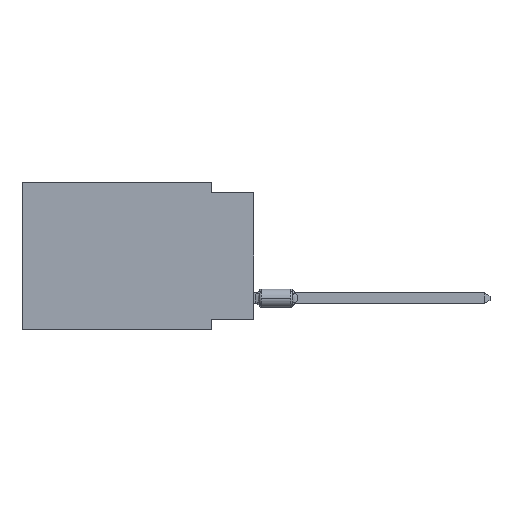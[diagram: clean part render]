
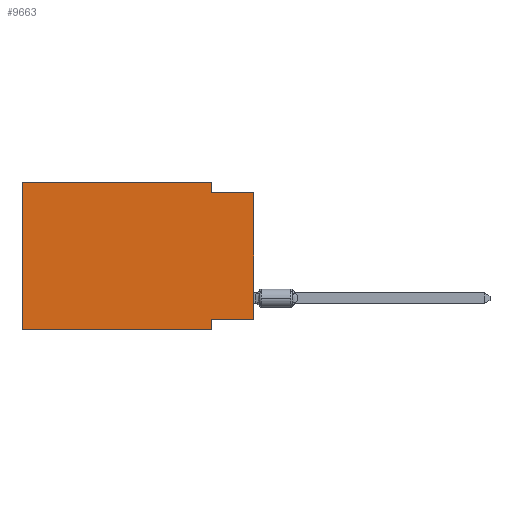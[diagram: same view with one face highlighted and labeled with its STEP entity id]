
A CAD part, left-side view. The second image highlights one B-rep face of the part: STEP entity #9663.
In plain terms, the highlighted planar face has unit normal (-1, 0, 0).
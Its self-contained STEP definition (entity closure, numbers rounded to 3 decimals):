
#119 = EDGE_CURVE ( 'NONE', #4076, #11084, #7150, .T. ) ;
#1149 = EDGE_CURVE ( 'NONE', #2157, #9634, #4121, .T. ) ;
#1265 = VECTOR ( 'NONE', #4323, 1000. ) ;
#1350 = DIRECTION ( 'NONE',  ( 0., 0., -1. ) ) ;
#1487 = LINE ( 'NONE', #12719, #3910 ) ;
#1554 = EDGE_CURVE ( 'NONE', #5131, #2082, #3403, .T. ) ;
#1648 = ORIENTED_EDGE ( 'NONE', *, *, #1554, .F. ) ;
#1771 = VECTOR ( 'NONE', #1350, 1000. ) ;
#2082 = VERTEX_POINT ( 'NONE', #5509 ) ;
#2157 = VERTEX_POINT ( 'NONE', #2670 ) ;
#2222 = ORIENTED_EDGE ( 'NONE', *, *, #9824, .T. ) ;
#2359 = ORIENTED_EDGE ( 'NONE', *, *, #119, .F. ) ;
#2578 = LINE ( 'NONE', #8451, #3247 ) ;
#2670 = CARTESIAN_POINT ( 'NONE',  ( 0., 13.97, -8.89 ) ) ;
#2773 = VECTOR ( 'NONE', #11607, 1000. ) ;
#3015 = ORIENTED_EDGE ( 'NONE', *, *, #6114, .F. ) ;
#3231 = LINE ( 'NONE', #10504, #1771 ) ;
#3247 = VECTOR ( 'NONE', #11606, 1000. ) ;
#3403 = LINE ( 'NONE', #7505, #2773 ) ;
#3701 = AXIS2_PLACEMENT_3D ( 'NONE', #9966, #6735, #7949 ) ;
#3910 = VECTOR ( 'NONE', #8354, 1000. ) ;
#4076 = VERTEX_POINT ( 'NONE', #4730 ) ;
#4086 = CARTESIAN_POINT ( 'NONE',  ( 0., 0., -8.255 ) ) ;
#4121 = LINE ( 'NONE', #11397, #1265 ) ;
#4323 = DIRECTION ( 'NONE',  ( 0., 0., 1. ) ) ;
#4683 = VECTOR ( 'NONE', #11817, 1000. ) ;
#4730 = CARTESIAN_POINT ( 'NONE',  ( 0., 2.54, -0.635 ) ) ;
#5131 = VERTEX_POINT ( 'NONE', #4086 ) ;
#5509 = CARTESIAN_POINT ( 'NONE',  ( 0., 2.54, -8.255 ) ) ;
#5958 = EDGE_CURVE ( 'NONE', #2157, #9488, #12956, .T. ) ;
#6114 = EDGE_CURVE ( 'NONE', #9634, #10293, #13154, .T. ) ;
#6343 = CARTESIAN_POINT ( 'NONE',  ( 0., 2.54, -8.89 ) ) ;
#6682 = ORIENTED_EDGE ( 'NONE', *, *, #1149, .F. ) ;
#6698 = ORIENTED_EDGE ( 'NONE', *, *, #9852, .F. ) ;
#6735 = DIRECTION ( 'NONE',  ( 1., 0., 0. ) ) ;
#7150 = LINE ( 'NONE', #8375, #8580 ) ;
#7209 = ORIENTED_EDGE ( 'NONE', *, *, #5958, .T. ) ;
#7229 = CARTESIAN_POINT ( 'NONE',  ( 0., 13.97, 0. ) ) ;
#7505 = CARTESIAN_POINT ( 'NONE',  ( 0., 0., -8.255 ) ) ;
#7733 = EDGE_LOOP ( 'NONE', ( #2222, #2359, #6698, #3015, #6682, #7209, #10249, #1648 ) ) ;
#7742 = FACE_OUTER_BOUND ( 'NONE', #7733, .T. ) ;
#7805 = CARTESIAN_POINT ( 'NONE',  ( 0., 13.97, 0. ) ) ;
#7949 = DIRECTION ( 'NONE',  ( 0., 0., -1. ) ) ;
#8354 = DIRECTION ( 'NONE',  ( 0., 0., 1. ) ) ;
#8375 = CARTESIAN_POINT ( 'NONE',  ( 0., 0., -0.635 ) ) ;
#8451 = CARTESIAN_POINT ( 'NONE',  ( 0., 2.54, -8.89 ) ) ;
#8580 = VECTOR ( 'NONE', #10448, 1000. ) ;
#8612 = EDGE_CURVE ( 'NONE', #2082, #9488, #2578, .T. ) ;
#8795 = CARTESIAN_POINT ( 'NONE',  ( 0., 2.54, 0. ) ) ;
#9488 = VERTEX_POINT ( 'NONE', #6343 ) ;
#9633 = VECTOR ( 'NONE', #10330, 1000. ) ;
#9634 = VERTEX_POINT ( 'NONE', #7805 ) ;
#9663 = ADVANCED_FACE ( 'NONE', ( #7742 ), #11981, .F. ) ;
#9824 = EDGE_CURVE ( 'NONE', #5131, #11084, #1487, .T. ) ;
#9852 = EDGE_CURVE ( 'NONE', #10293, #4076, #3231, .T. ) ;
#9966 = CARTESIAN_POINT ( 'NONE',  ( 0., 13.97, 0. ) ) ;
#10249 = ORIENTED_EDGE ( 'NONE', *, *, #8612, .F. ) ;
#10293 = VERTEX_POINT ( 'NONE', #8795 ) ;
#10330 = DIRECTION ( 'NONE',  ( 0., -1., 0. ) ) ;
#10448 = DIRECTION ( 'NONE',  ( 0., -1., 0. ) ) ;
#10504 = CARTESIAN_POINT ( 'NONE',  ( 0., 2.54, 0. ) ) ;
#11072 = CARTESIAN_POINT ( 'NONE',  ( 0., 13.97, -8.89 ) ) ;
#11084 = VERTEX_POINT ( 'NONE', #12914 ) ;
#11397 = CARTESIAN_POINT ( 'NONE',  ( 0., 13.97, 0. ) ) ;
#11606 = DIRECTION ( 'NONE',  ( 0., 0., -1. ) ) ;
#11607 = DIRECTION ( 'NONE',  ( 0., 1., 0. ) ) ;
#11817 = DIRECTION ( 'NONE',  ( 0., -1., 0. ) ) ;
#11981 = PLANE ( 'NONE',  #3701 ) ;
#12719 = CARTESIAN_POINT ( 'NONE',  ( 0., 0., 0. ) ) ;
#12914 = CARTESIAN_POINT ( 'NONE',  ( 0., 0., -0.635 ) ) ;
#12956 = LINE ( 'NONE', #11072, #4683 ) ;
#13154 = LINE ( 'NONE', #7229, #9633 ) ;
